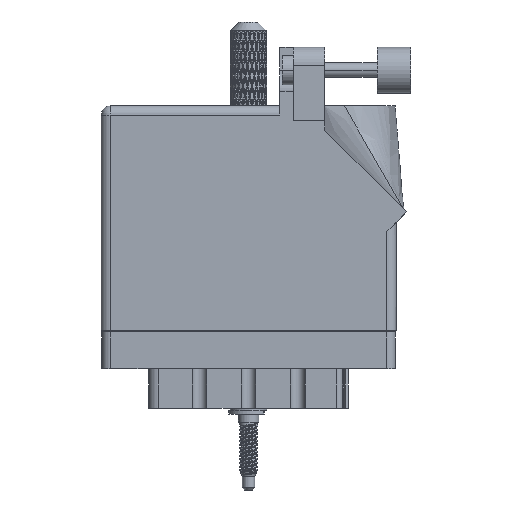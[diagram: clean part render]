
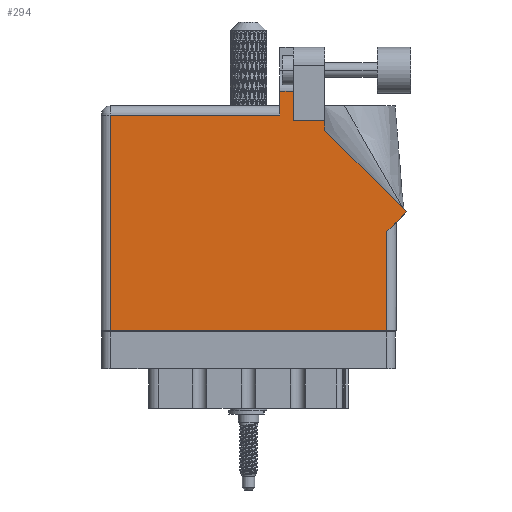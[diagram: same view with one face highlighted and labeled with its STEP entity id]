
A CAD part, front view. The second image highlights one B-rep face of the part: STEP entity #294.
In plain terms, the highlighted face is planar.
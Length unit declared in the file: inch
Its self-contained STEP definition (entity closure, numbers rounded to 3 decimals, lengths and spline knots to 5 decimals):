
#294 = ADVANCED_FACE ( 'NONE', ( #98213 ), #25967, .F. ) ;
#867 = CARTESIAN_POINT ( 'NONE',  ( 1.524, 1.36442, 0. ) ) ;
#972 = CARTESIAN_POINT ( 'NONE',  ( 0., 1.53, 0. ) ) ;
#3190 = VERTEX_POINT ( 'NONE', #39095 ) ;
#10575 = LINE ( 'NONE', #51868, #45000 ) ;
#11105 = DIRECTION ( 'NONE',  ( -1., 0., 0. ) ) ;
#13042 = EDGE_LOOP ( 'NONE', ( #103184, #36502, #65506, #51944, #80967, #19406, #46557, #101169, #49991, #84850, #40983 ) ) ;
#14665 = VECTOR ( 'NONE', #60095, 39.37008 ) ;
#17031 = VECTOR ( 'NONE', #88485, 39.37008 ) ;
#17435 = VERTEX_POINT ( 'NONE', #26304 ) ;
#19406 = ORIENTED_EDGE ( 'NONE', *, *, #55200, .T. ) ;
#21442 = VECTOR ( 'NONE', #66235, 39.37008 ) ;
#22458 = CARTESIAN_POINT ( 'NONE',  ( 1.948, 0., 0. ) ) ;
#24209 = CARTESIAN_POINT ( 'NONE',  ( 2.08071, 0.80771, 0. ) ) ;
#24349 = DIRECTION ( 'NONE',  ( 0., 0., -1. ) ) ;
#25967 = PLANE ( 'NONE',  #78926 ) ;
#26231 = VERTEX_POINT ( 'NONE', #867 ) ;
#26304 = CARTESIAN_POINT ( 'NONE',  ( 1.217, 1.468, 0. ) ) ;
#28161 = LINE ( 'NONE', #50482, #40557 ) ;
#28176 = VERTEX_POINT ( 'NONE', #53685 ) ;
#28511 = LINE ( 'NONE', #76864, #67362 ) ;
#28617 = VECTOR ( 'NONE', #72853, 39.37008 ) ;
#35089 = CARTESIAN_POINT ( 'NONE',  ( 1.948, 0.737, 0. ) ) ;
#36502 = ORIENTED_EDGE ( 'NONE', *, *, #66906, .T. ) ;
#37894 = VERTEX_POINT ( 'NONE', #79919 ) ;
#39095 = CARTESIAN_POINT ( 'NONE',  ( 1.217, 1.6315, 0. ) ) ;
#39651 = CARTESIAN_POINT ( 'NONE',  ( 1.64177, 1.6315, 0. ) ) ;
#39709 = CARTESIAN_POINT ( 'NONE',  ( 1.524, 1.36442, 0. ) ) ;
#40251 = VERTEX_POINT ( 'NONE', #57874 ) ;
#40557 = VECTOR ( 'NONE', #83613, 39.37008 ) ;
#40983 = ORIENTED_EDGE ( 'NONE', *, *, #83381, .T. ) ;
#42196 = CARTESIAN_POINT ( 'NONE',  ( 1.311, 1.43, 0. ) ) ;
#42543 = VECTOR ( 'NONE', #58377, 39.37008 ) ;
#45000 = VECTOR ( 'NONE', #11105, 39.37008 ) ;
#45841 = VERTEX_POINT ( 'NONE', #100621 ) ;
#46139 = LINE ( 'NONE', #89029, #17031 ) ;
#46557 = ORIENTED_EDGE ( 'NONE', *, *, #77681, .T. ) ;
#49004 = LINE ( 'NONE', #87179, #70234 ) ;
#49991 = ORIENTED_EDGE ( 'NONE', *, *, #56173, .T. ) ;
#50482 = CARTESIAN_POINT ( 'NONE',  ( 1.217, 1.53, 0. ) ) ;
#50821 = VERTEX_POINT ( 'NONE', #22458 ) ;
#50926 = DIRECTION ( 'NONE',  ( -1., 0., 0. ) ) ;
#51537 = CARTESIAN_POINT ( 'NONE',  ( 0.062, 1.468, 0. ) ) ;
#51868 = CARTESIAN_POINT ( 'NONE',  ( 1.524, 1.43, 0. ) ) ;
#51944 = ORIENTED_EDGE ( 'NONE', *, *, #58667, .T. ) ;
#53685 = CARTESIAN_POINT ( 'NONE',  ( 1.311, 1.6315, 0. ) ) ;
#55200 = EDGE_CURVE ( 'NONE', #45841, #50821, #49004, .T. ) ;
#56173 = EDGE_CURVE ( 'NONE', #61479, #26231, #98600, .T. ) ;
#56344 = CARTESIAN_POINT ( 'NONE',  ( 1.524, 1.43, 0. ) ) ;
#57447 = EDGE_CURVE ( 'NONE', #40251, #61479, #75123, .T. ) ;
#57730 = DIRECTION ( 'NONE',  ( 0.707, 0.707, 0. ) ) ;
#57874 = CARTESIAN_POINT ( 'NONE',  ( 1.948, 0.675, 0. ) ) ;
#58377 = DIRECTION ( 'NONE',  ( -0.707, 0.707, 0. ) ) ;
#58380 = VECTOR ( 'NONE', #68204, 39.37008 ) ;
#58667 = EDGE_CURVE ( 'NONE', #17435, #59861, #46139, .T. ) ;
#59861 = VERTEX_POINT ( 'NONE', #51537 ) ;
#60095 = DIRECTION ( 'NONE',  ( 0., 1., 0. ) ) ;
#61479 = VERTEX_POINT ( 'NONE', #66557 ) ;
#65362 = CARTESIAN_POINT ( 'NONE',  ( 2.01, 0.737, 0. ) ) ;
#65506 = ORIENTED_EDGE ( 'NONE', *, *, #67042, .T. ) ;
#66235 = DIRECTION ( 'NONE',  ( -1., 0., 0. ) ) ;
#66557 = CARTESIAN_POINT ( 'NONE',  ( 2.08071, 0.80771, 0. ) ) ;
#66906 = EDGE_CURVE ( 'NONE', #28176, #3190, #91757, .T. ) ;
#67042 = EDGE_CURVE ( 'NONE', #3190, #17435, #28161, .T. ) ;
#67345 = VERTEX_POINT ( 'NONE', #56344 ) ;
#67362 = VECTOR ( 'NONE', #94766, 39.37008 ) ;
#67713 = LINE ( 'NONE', #42196, #14665 ) ;
#68204 = DIRECTION ( 'NONE',  ( 0., 1., 0. ) ) ;
#70234 = VECTOR ( 'NONE', #82131, 39.37008 ) ;
#72853 = DIRECTION ( 'NONE',  ( 0., 1., 0. ) ) ;
#73166 = EDGE_CURVE ( 'NONE', #37894, #28176, #67713, .T. ) ;
#75123 = LINE ( 'NONE', #65362, #79048 ) ;
#76343 = LINE ( 'NONE', #35089, #58380 ) ;
#76864 = CARTESIAN_POINT ( 'NONE',  ( 0.062, 0., 0. ) ) ;
#77681 = EDGE_CURVE ( 'NONE', #50821, #40251, #76343, .T. ) ;
#78926 = AXIS2_PLACEMENT_3D ( 'NONE', #972, #24349, #50926 ) ;
#79048 = VECTOR ( 'NONE', #57730, 39.37008 ) ;
#79919 = CARTESIAN_POINT ( 'NONE',  ( 1.311, 1.43, 0. ) ) ;
#80967 = ORIENTED_EDGE ( 'NONE', *, *, #84721, .T. ) ;
#80984 = LINE ( 'NONE', #39709, #28617 ) ;
#82131 = DIRECTION ( 'NONE',  ( 1., 0., 0. ) ) ;
#83381 = EDGE_CURVE ( 'NONE', #67345, #37894, #10575, .T. ) ;
#83613 = DIRECTION ( 'NONE',  ( 0., -1., 0. ) ) ;
#84721 = EDGE_CURVE ( 'NONE', #59861, #45841, #28511, .T. ) ;
#84850 = ORIENTED_EDGE ( 'NONE', *, *, #98847, .T. ) ;
#87179 = CARTESIAN_POINT ( 'NONE',  ( 0., 0., 0. ) ) ;
#88485 = DIRECTION ( 'NONE',  ( -1., 0., 0. ) ) ;
#89029 = CARTESIAN_POINT ( 'NONE',  ( 0., 1.468, 0. ) ) ;
#91757 = LINE ( 'NONE', #39651, #21442 ) ;
#94766 = DIRECTION ( 'NONE',  ( 0., -1., 0. ) ) ;
#98213 = FACE_OUTER_BOUND ( 'NONE', #13042, .T. ) ;
#98600 = LINE ( 'NONE', #24209, #42543 ) ;
#98847 = EDGE_CURVE ( 'NONE', #26231, #67345, #80984, .T. ) ;
#100621 = CARTESIAN_POINT ( 'NONE',  ( 0.062, 0., 0. ) ) ;
#101169 = ORIENTED_EDGE ( 'NONE', *, *, #57447, .T. ) ;
#103184 = ORIENTED_EDGE ( 'NONE', *, *, #73166, .T. ) ;
